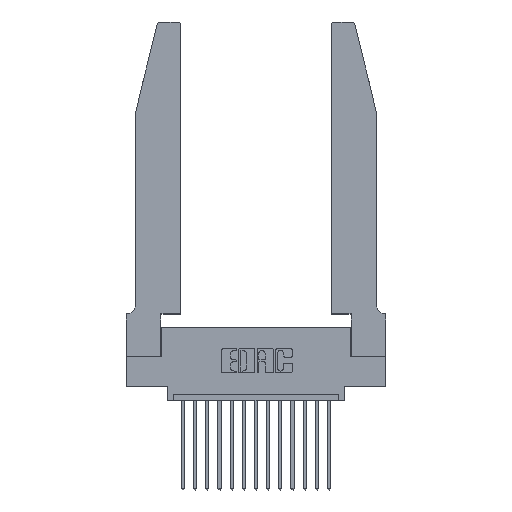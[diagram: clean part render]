
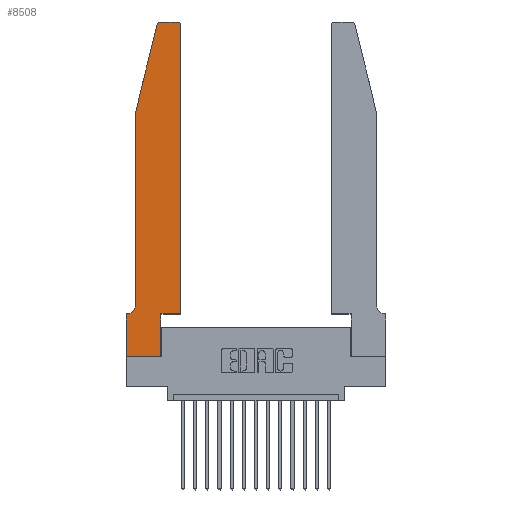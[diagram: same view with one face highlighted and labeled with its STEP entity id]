
A CAD part, top view. The second image highlights one B-rep face of the part: STEP entity #8508.
In plain terms, the highlighted planar face has unit normal (0, 0, 1).
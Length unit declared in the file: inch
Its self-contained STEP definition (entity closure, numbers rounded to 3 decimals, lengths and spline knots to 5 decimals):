
#271 = ORIENTED_EDGE ( 'NONE', *, *, #13027, .T. ) ;
#454 = DIRECTION ( 'NONE',  ( 0., -1., 0. ) ) ;
#581 = CARTESIAN_POINT ( 'NONE',  ( 0.2865, 0.35, 0.37 ) ) ;
#1274 = LINE ( 'NONE', #3741, #10050 ) ;
#1318 = PLANE ( 'NONE',  #11889 ) ;
#1417 = CARTESIAN_POINT ( 'NONE',  ( 0.284, 2.72, 0.37 ) ) ;
#1426 = CARTESIAN_POINT ( 'NONE',  ( 0.2865, 0., 0.37 ) ) ;
#1465 = DIRECTION ( 'NONE',  ( -0.239, -0.971, 0. ) ) ;
#1650 = VECTOR ( 'NONE', #8410, 39.37008 ) ;
#1764 = DIRECTION ( 'NONE',  ( -1., 0., 0. ) ) ;
#2014 = VERTEX_POINT ( 'NONE', #11836 ) ;
#2120 = LINE ( 'NONE', #12956, #1650 ) ;
#2540 = EDGE_CURVE ( 'NONE', #5983, #10054, #7776, .T. ) ;
#2768 = VERTEX_POINT ( 'NONE', #8929 ) ;
#3017 = VECTOR ( 'NONE', #1764, 39.37008 ) ;
#3072 = FACE_OUTER_BOUND ( 'NONE', #7244, .T. ) ;
#3741 = CARTESIAN_POINT ( 'NONE',  ( 0.4505, 0.35, 0.37 ) ) ;
#3780 = ORIENTED_EDGE ( 'NONE', *, *, #12973, .T. ) ;
#3936 = CARTESIAN_POINT ( 'NONE',  ( 0., 0.35, 0.37 ) ) ;
#4277 = EDGE_CURVE ( 'NONE', #13895, #12642, #11142, .T. ) ;
#4373 = CIRCLE ( 'NONE', #17693, 0.03 ) ;
#4459 = DIRECTION ( 'NONE',  ( 1., 0., 0. ) ) ;
#4488 = AXIS2_PLACEMENT_3D ( 'NONE', #5903, #15916, #12820 ) ;
#4522 = EDGE_CURVE ( 'NONE', #2768, #5983, #12914, .T. ) ;
#4701 = CARTESIAN_POINT ( 'NONE',  ( 0.25487, 2.72718, 0.37 ) ) ;
#4958 = EDGE_CURVE ( 'NONE', #15785, #2014, #8155, .T. ) ;
#4975 = CARTESIAN_POINT ( 'NONE',  ( 0.2865, 0.35, 0.37 ) ) ;
#5016 = LINE ( 'NONE', #15566, #10685 ) ;
#5065 = CARTESIAN_POINT ( 'NONE',  ( 0.4205, 2.72, 0.37 ) ) ;
#5245 = DIRECTION ( 'NONE',  ( 0., 1., 0. ) ) ;
#5265 = CIRCLE ( 'NONE', #4488, 0.07 ) ;
#5528 = LINE ( 'NONE', #15072, #12518 ) ;
#5828 = DIRECTION ( 'NONE',  ( -1., 0., 0. ) ) ;
#5903 = CARTESIAN_POINT ( 'NONE',  ( 0.0055, 0.42, 0.37 ) ) ;
#5932 = DIRECTION ( 'NONE',  ( 0., 0., 1. ) ) ;
#5983 = VERTEX_POINT ( 'NONE', #11730 ) ;
#6473 = ORIENTED_EDGE ( 'NONE', *, *, #4958, .T. ) ;
#7244 = EDGE_LOOP ( 'NONE', ( #9601, #7974, #3780, #8607, #17501, #18462, #6473, #13977, #16317, #271, #12412, #13019 ) ) ;
#7257 = VECTOR ( 'NONE', #5828, 39.37008 ) ;
#7776 = CIRCLE ( 'NONE', #14685, 0.03 ) ;
#7974 = ORIENTED_EDGE ( 'NONE', *, *, #2540, .T. ) ;
#8155 = LINE ( 'NONE', #13318, #9972 ) ;
#8408 = CARTESIAN_POINT ( 'NONE',  ( 0.4505, 0.35, 0.37 ) ) ;
#8410 = DIRECTION ( 'NONE',  ( 1., 0., 0. ) ) ;
#8508 = ADVANCED_FACE ( 'NONE', ( #3072 ), #1318, .T. ) ;
#8543 = EDGE_CURVE ( 'NONE', #16997, #12595, #5528, .T. ) ;
#8607 = ORIENTED_EDGE ( 'NONE', *, *, #8543, .T. ) ;
#8929 = CARTESIAN_POINT ( 'NONE',  ( 0.4205, 2.75, 0.37 ) ) ;
#8964 = EDGE_CURVE ( 'NONE', #9754, #12712, #1274, .T. ) ;
#9601 = ORIENTED_EDGE ( 'NONE', *, *, #4522, .T. ) ;
#9727 = LINE ( 'NONE', #15995, #11322 ) ;
#9754 = VERTEX_POINT ( 'NONE', #8408 ) ;
#9972 = VECTOR ( 'NONE', #454, 39.37008 ) ;
#10050 = VECTOR ( 'NONE', #5245, 39.37008 ) ;
#10054 = VERTEX_POINT ( 'NONE', #4701 ) ;
#10543 = DIRECTION ( 'NONE',  ( 1., 0., 0. ) ) ;
#10637 = DIRECTION ( 'NONE',  ( 0., 0., 1. ) ) ;
#10685 = VECTOR ( 'NONE', #1465, 39.37008 ) ;
#11142 = LINE ( 'NONE', #581, #16914 ) ;
#11322 = VECTOR ( 'NONE', #4459, 39.37008 ) ;
#11512 = CARTESIAN_POINT ( 'NONE',  ( 0., 0.35, 0.37 ) ) ;
#11730 = CARTESIAN_POINT ( 'NONE',  ( 0.284, 2.75, 0.37 ) ) ;
#11836 = CARTESIAN_POINT ( 'NONE',  ( 0., 0., 0.37 ) ) ;
#11840 = CARTESIAN_POINT ( 'NONE',  ( 0.2605, 2.75, 0.37 ) ) ;
#11889 = AXIS2_PLACEMENT_3D ( 'NONE', #11512, #12946, #14364 ) ;
#12083 = CARTESIAN_POINT ( 'NONE',  ( 0.4505, 2.72, 0.37 ) ) ;
#12412 = ORIENTED_EDGE ( 'NONE', *, *, #8964, .T. ) ;
#12518 = VECTOR ( 'NONE', #15324, 39.37008 ) ;
#12595 = VERTEX_POINT ( 'NONE', #16370 ) ;
#12642 = VERTEX_POINT ( 'NONE', #4975 ) ;
#12712 = VERTEX_POINT ( 'NONE', #12083 ) ;
#12820 = DIRECTION ( 'NONE',  ( -1., 0., 0. ) ) ;
#12914 = LINE ( 'NONE', #11840, #3017 ) ;
#12946 = DIRECTION ( 'NONE',  ( 0., 0., 1. ) ) ;
#12956 = CARTESIAN_POINT ( 'NONE',  ( 0.4505, 0.35, 0.37 ) ) ;
#12973 = EDGE_CURVE ( 'NONE', #10054, #16997, #5016, .T. ) ;
#13019 = ORIENTED_EDGE ( 'NONE', *, *, #17424, .T. ) ;
#13027 = EDGE_CURVE ( 'NONE', #12642, #9754, #2120, .T. ) ;
#13087 = EDGE_CURVE ( 'NONE', #2014, #13895, #9727, .T. ) ;
#13318 = CARTESIAN_POINT ( 'NONE',  ( 0., 0., 0.37 ) ) ;
#13895 = VERTEX_POINT ( 'NONE', #1426 ) ;
#13977 = ORIENTED_EDGE ( 'NONE', *, *, #13087, .T. ) ;
#14235 = LINE ( 'NONE', #14294, #7257 ) ;
#14294 = CARTESIAN_POINT ( 'NONE',  ( 0.0755, 0.35, 0.37 ) ) ;
#14305 = CARTESIAN_POINT ( 'NONE',  ( 0.0755, 2., 0.37 ) ) ;
#14364 = DIRECTION ( 'NONE',  ( 1., 0., 0. ) ) ;
#14685 = AXIS2_PLACEMENT_3D ( 'NONE', #1417, #5932, #10543 ) ;
#14779 = DIRECTION ( 'NONE',  ( 0., 1., 0. ) ) ;
#15072 = CARTESIAN_POINT ( 'NONE',  ( 0.0755, 2., 0.37 ) ) ;
#15324 = DIRECTION ( 'NONE',  ( 0., -1., 0. ) ) ;
#15566 = CARTESIAN_POINT ( 'NONE',  ( 0.0755, 2., 0.37 ) ) ;
#15785 = VERTEX_POINT ( 'NONE', #3936 ) ;
#15916 = DIRECTION ( 'NONE',  ( 0., 0., -1. ) ) ;
#15995 = CARTESIAN_POINT ( 'NONE',  ( 0., 0., 0.37 ) ) ;
#16055 = VERTEX_POINT ( 'NONE', #17395 ) ;
#16317 = ORIENTED_EDGE ( 'NONE', *, *, #4277, .T. ) ;
#16370 = CARTESIAN_POINT ( 'NONE',  ( 0.0755, 0.42, 0.37 ) ) ;
#16532 = DIRECTION ( 'NONE',  ( 1., 0., 0. ) ) ;
#16914 = VECTOR ( 'NONE', #14779, 39.37008 ) ;
#16997 = VERTEX_POINT ( 'NONE', #14305 ) ;
#17097 = EDGE_CURVE ( 'NONE', #12595, #16055, #5265, .T. ) ;
#17395 = CARTESIAN_POINT ( 'NONE',  ( 0.0055, 0.35, 0.37 ) ) ;
#17424 = EDGE_CURVE ( 'NONE', #12712, #2768, #4373, .T. ) ;
#17501 = ORIENTED_EDGE ( 'NONE', *, *, #17097, .T. ) ;
#17654 = EDGE_CURVE ( 'NONE', #16055, #15785, #14235, .T. ) ;
#17693 = AXIS2_PLACEMENT_3D ( 'NONE', #5065, #10637, #16532 ) ;
#18462 = ORIENTED_EDGE ( 'NONE', *, *, #17654, .T. ) ;
